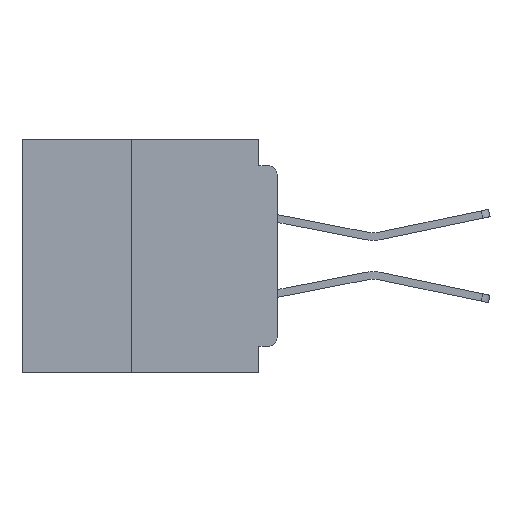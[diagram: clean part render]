
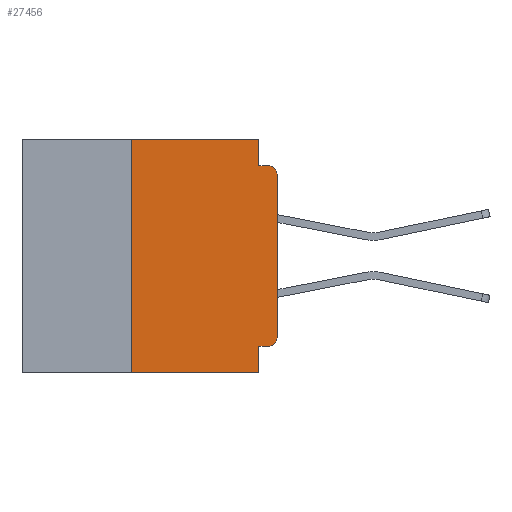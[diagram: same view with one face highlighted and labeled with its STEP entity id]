
A CAD part, left-side view. The second image highlights one B-rep face of the part: STEP entity #27456.
In plain terms, the highlighted planar face has unit normal (-1, 0, 0).
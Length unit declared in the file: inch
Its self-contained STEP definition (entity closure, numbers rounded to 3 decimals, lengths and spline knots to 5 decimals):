
#202 = ORIENTED_EDGE ( 'NONE', *, *, #1534, .F. ) ;
#669 = LINE ( 'NONE', #23060, #50226 ) ;
#951 = CARTESIAN_POINT ( 'NONE',  ( 0., 0.437, 0. ) ) ;
#1534 = EDGE_CURVE ( 'NONE', #49677, #15854, #8393, .T. ) ;
#1600 = DIRECTION ( 'NONE',  ( 0., 0., 1. ) ) ;
#5540 = PLANE ( 'NONE',  #37292 ) ;
#6534 = VECTOR ( 'NONE', #18013, 39.37008 ) ;
#7127 = ORIENTED_EDGE ( 'NONE', *, *, #15797, .F. ) ;
#8393 = LINE ( 'NONE', #39498, #41603 ) ;
#8691 = ORIENTED_EDGE ( 'NONE', *, *, #8806, .T. ) ;
#8747 = ORIENTED_EDGE ( 'NONE', *, *, #50565, .F. ) ;
#8806 = EDGE_CURVE ( 'NONE', #55207, #13695, #8833, .T. ) ;
#8833 = LINE ( 'NONE', #33297, #31519 ) ;
#8974 = LINE ( 'NONE', #52526, #31640 ) ;
#9121 = DIRECTION ( 'NONE',  ( -1., 0., 0. ) ) ;
#9431 = VERTEX_POINT ( 'NONE', #53595 ) ;
#10097 = DIRECTION ( 'NONE',  ( 0., 0., -1. ) ) ;
#10159 = FACE_OUTER_BOUND ( 'NONE', #44653, .T. ) ;
#11320 = CARTESIAN_POINT ( 'NONE',  ( 0., 0.015, -0.045 ) ) ;
#11450 = VERTEX_POINT ( 'NONE', #18752 ) ;
#13322 = DIRECTION ( 'NONE',  ( -1., 0., 0. ) ) ;
#13695 = VERTEX_POINT ( 'NONE', #53920 ) ;
#15749 = VECTOR ( 'NONE', #49142, 39.37008 ) ;
#15797 = EDGE_CURVE ( 'NONE', #42036, #11450, #51719, .T. ) ;
#15854 = VERTEX_POINT ( 'NONE', #40264 ) ;
#15962 = CARTESIAN_POINT ( 'NONE',  ( 0., 0.015, -0.355 ) ) ;
#16028 = AXIS2_PLACEMENT_3D ( 'NONE', #36154, #9121, #40738 ) ;
#17399 = VECTOR ( 'NONE', #52878, 39.37008 ) ;
#18013 = DIRECTION ( 'NONE',  ( 0., 0., 1. ) ) ;
#18752 = CARTESIAN_POINT ( 'NONE',  ( 0., 0.031, -0.045 ) ) ;
#18816 = LINE ( 'NONE', #25937, #17399 ) ;
#20350 = EDGE_CURVE ( 'NONE', #58277, #42036, #54558, .T. ) ;
#20909 = EDGE_CURVE ( 'NONE', #13695, #32492, #24942, .T. ) ;
#21045 = DIRECTION ( 'NONE',  ( 0., -1., 0. ) ) ;
#22730 = EDGE_CURVE ( 'NONE', #49677, #55207, #32396, .T. ) ;
#23060 = CARTESIAN_POINT ( 'NONE',  ( 0., 0., -0.045 ) ) ;
#23247 = VERTEX_POINT ( 'NONE', #44396 ) ;
#24593 = DIRECTION ( 'NONE',  ( 0., -1., 0. ) ) ;
#24942 = CIRCLE ( 'NONE', #35136, 0.015 ) ;
#25937 = CARTESIAN_POINT ( 'NONE',  ( 0., 0.031, -0.4 ) ) ;
#27456 = ADVANCED_FACE ( 'NONE', ( #10159 ), #5540, .F. ) ;
#29102 = CARTESIAN_POINT ( 'NONE',  ( 0., 0.437, 0. ) ) ;
#29208 = VECTOR ( 'NONE', #24593, 39.37008 ) ;
#31519 = VECTOR ( 'NONE', #1600, 39.37008 ) ;
#31640 = VECTOR ( 'NONE', #21045, 39.37008 ) ;
#32396 = CIRCLE ( 'NONE', #16028, 0.015 ) ;
#32402 = CARTESIAN_POINT ( 'NONE',  ( 0., 0.25, 0. ) ) ;
#32492 = VERTEX_POINT ( 'NONE', #11320 ) ;
#32989 = ORIENTED_EDGE ( 'NONE', *, *, #20350, .F. ) ;
#33297 = CARTESIAN_POINT ( 'NONE',  ( 0., 0., 0. ) ) ;
#35136 = AXIS2_PLACEMENT_3D ( 'NONE', #40331, #13322, #44840 ) ;
#35874 = EDGE_CURVE ( 'NONE', #11450, #32492, #669, .T. ) ;
#36154 = CARTESIAN_POINT ( 'NONE',  ( 0., 0.015, -0.34 ) ) ;
#37292 = AXIS2_PLACEMENT_3D ( 'NONE', #951, #41509, #10097 ) ;
#38931 = ORIENTED_EDGE ( 'NONE', *, *, #22730, .T. ) ;
#39449 = CARTESIAN_POINT ( 'NONE',  ( 0., 0., -0.34 ) ) ;
#39498 = CARTESIAN_POINT ( 'NONE',  ( 0., 0., -0.355 ) ) ;
#40264 = CARTESIAN_POINT ( 'NONE',  ( 0., 0.031, -0.355 ) ) ;
#40331 = CARTESIAN_POINT ( 'NONE',  ( 0., 0.015, -0.06 ) ) ;
#40738 = DIRECTION ( 'NONE',  ( 0., 0., -1. ) ) ;
#41152 = LINE ( 'NONE', #44953, #6534 ) ;
#41399 = ORIENTED_EDGE ( 'NONE', *, *, #35874, .F. ) ;
#41509 = DIRECTION ( 'NONE',  ( 1., 0., 0. ) ) ;
#41603 = VECTOR ( 'NONE', #48375, 39.37008 ) ;
#42036 = VERTEX_POINT ( 'NONE', #48925 ) ;
#44396 = CARTESIAN_POINT ( 'NONE',  ( 0., 0.25, -0.4 ) ) ;
#44583 = CARTESIAN_POINT ( 'NONE',  ( 0., 0.031, 0. ) ) ;
#44653 = EDGE_LOOP ( 'NONE', ( #8691, #48072, #41399, #7127, #32989, #53389, #56776, #8747, #202, #38931 ) ) ;
#44840 = DIRECTION ( 'NONE',  ( 0., 0., -1. ) ) ;
#44953 = CARTESIAN_POINT ( 'NONE',  ( 0., 0.25, -0.4 ) ) ;
#48072 = ORIENTED_EDGE ( 'NONE', *, *, #20909, .T. ) ;
#48375 = DIRECTION ( 'NONE',  ( 0., 1., 0. ) ) ;
#48925 = CARTESIAN_POINT ( 'NONE',  ( 0., 0.031, 0. ) ) ;
#49142 = DIRECTION ( 'NONE',  ( 0., 0., -1. ) ) ;
#49677 = VERTEX_POINT ( 'NONE', #15962 ) ;
#50008 = DIRECTION ( 'NONE',  ( 0., -1., 0. ) ) ;
#50226 = VECTOR ( 'NONE', #50008, 39.37008 ) ;
#50565 = EDGE_CURVE ( 'NONE', #15854, #9431, #18816, .T. ) ;
#51719 = LINE ( 'NONE', #44583, #15749 ) ;
#52526 = CARTESIAN_POINT ( 'NONE',  ( 0., 0.437, -0.4 ) ) ;
#52574 = EDGE_CURVE ( 'NONE', #23247, #58277, #41152, .T. ) ;
#52878 = DIRECTION ( 'NONE',  ( 0., 0., -1. ) ) ;
#53389 = ORIENTED_EDGE ( 'NONE', *, *, #52574, .F. ) ;
#53595 = CARTESIAN_POINT ( 'NONE',  ( 0., 0.031, -0.4 ) ) ;
#53920 = CARTESIAN_POINT ( 'NONE',  ( 0., 0., -0.06 ) ) ;
#54558 = LINE ( 'NONE', #29102, #29208 ) ;
#55207 = VERTEX_POINT ( 'NONE', #39449 ) ;
#56100 = EDGE_CURVE ( 'NONE', #23247, #9431, #8974, .T. ) ;
#56776 = ORIENTED_EDGE ( 'NONE', *, *, #56100, .T. ) ;
#58277 = VERTEX_POINT ( 'NONE', #32402 ) ;
